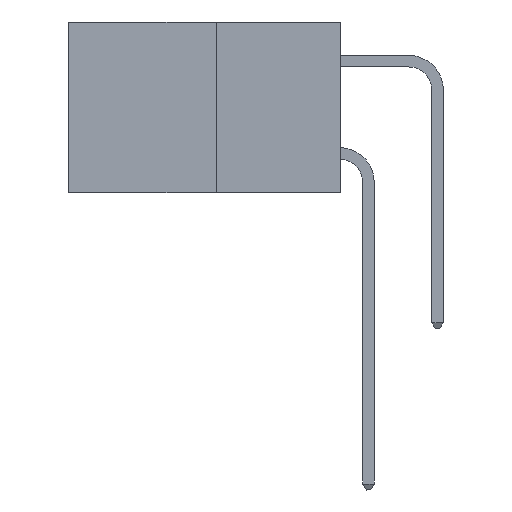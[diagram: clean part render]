
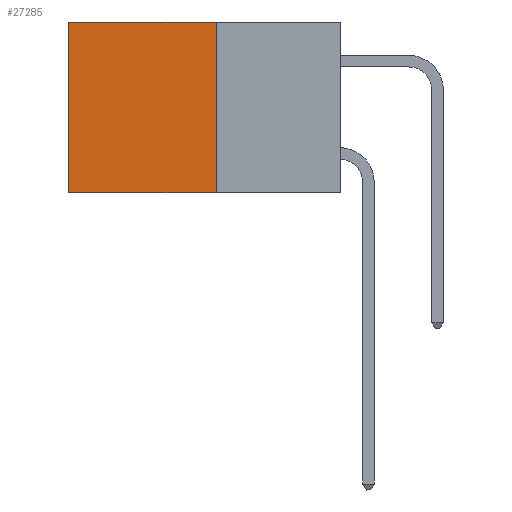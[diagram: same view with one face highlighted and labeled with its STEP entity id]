
A CAD part, left-side view. The second image highlights one B-rep face of the part: STEP entity #27285.
In plain terms, the highlighted planar face has unit normal (-1, 0, 0).
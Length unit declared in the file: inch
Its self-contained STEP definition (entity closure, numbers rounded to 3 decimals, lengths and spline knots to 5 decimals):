
#308 = EDGE_CURVE ( 'NONE', #3579, #23848, #25702, .T. ) ;
#497 = CARTESIAN_POINT ( 'NONE',  ( 0.277, 0.27, -0.37 ) ) ;
#586 = DIRECTION ( 'NONE',  ( 0., 0., -1. ) ) ;
#627 = VERTEX_POINT ( 'NONE', #2483 ) ;
#2220 = VERTEX_POINT ( 'NONE', #6440 ) ;
#2483 = CARTESIAN_POINT ( 'NONE',  ( 0.277, 0.27, -0.37 ) ) ;
#3579 = VERTEX_POINT ( 'NONE', #5254 ) ;
#3881 = FACE_OUTER_BOUND ( 'NONE', #5830, .T. ) ;
#5235 = VECTOR ( 'NONE', #22292, 39.37008 ) ;
#5254 = CARTESIAN_POINT ( 'NONE',  ( 0.277, 0.59, 0. ) ) ;
#5830 = EDGE_LOOP ( 'NONE', ( #16562, #5943, #12216, #7272 ) ) ;
#5943 = ORIENTED_EDGE ( 'NONE', *, *, #9719, .F. ) ;
#6200 = CARTESIAN_POINT ( 'NONE',  ( 0.277, 0.27, -0.37 ) ) ;
#6440 = CARTESIAN_POINT ( 'NONE',  ( 0.277, 0.27, 0. ) ) ;
#7272 = ORIENTED_EDGE ( 'NONE', *, *, #8550, .T. ) ;
#8313 = DIRECTION ( 'NONE',  ( 0., 0., -1. ) ) ;
#8550 = EDGE_CURVE ( 'NONE', #2220, #3579, #26975, .T. ) ;
#8912 = VECTOR ( 'NONE', #22418, 39.37008 ) ;
#9719 = EDGE_CURVE ( 'NONE', #627, #23848, #11475, .T. ) ;
#11311 = VECTOR ( 'NONE', #8313, 39.37008 ) ;
#11475 = LINE ( 'NONE', #24279, #5235 ) ;
#12216 = ORIENTED_EDGE ( 'NONE', *, *, #14883, .F. ) ;
#13245 = DIRECTION ( 'NONE',  ( 1., 0., 0. ) ) ;
#14883 = EDGE_CURVE ( 'NONE', #2220, #627, #22524, .T. ) ;
#16361 = AXIS2_PLACEMENT_3D ( 'NONE', #497, #13245, #586 ) ;
#16562 = ORIENTED_EDGE ( 'NONE', *, *, #308, .T. ) ;
#16862 = DIRECTION ( 'NONE',  ( 0., 1., 0. ) ) ;
#18892 = CARTESIAN_POINT ( 'NONE',  ( 0.277, 0.27, 0. ) ) ;
#21414 = VECTOR ( 'NONE', #16862, 39.37008 ) ;
#22292 = DIRECTION ( 'NONE',  ( 0., 1., 0. ) ) ;
#22418 = DIRECTION ( 'NONE',  ( 0., 0., -1. ) ) ;
#22524 = LINE ( 'NONE', #6200, #11311 ) ;
#23848 = VERTEX_POINT ( 'NONE', #23882 ) ;
#23882 = CARTESIAN_POINT ( 'NONE',  ( 0.277, 0.59, -0.37 ) ) ;
#24279 = CARTESIAN_POINT ( 'NONE',  ( 0.277, 0.27, -0.37 ) ) ;
#24335 = CARTESIAN_POINT ( 'NONE',  ( 0.277, 0.59, -0.37 ) ) ;
#25702 = LINE ( 'NONE', #24335, #8912 ) ;
#25818 = PLANE ( 'NONE',  #16361 ) ;
#26975 = LINE ( 'NONE', #18892, #21414 ) ;
#27285 = ADVANCED_FACE ( 'NONE', ( #3881 ), #25818, .F. ) ;
